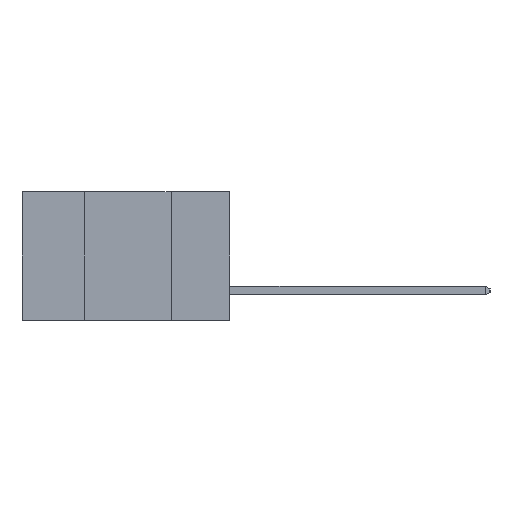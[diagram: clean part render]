
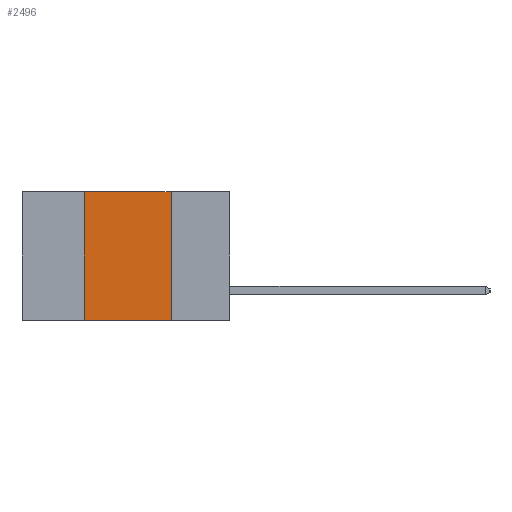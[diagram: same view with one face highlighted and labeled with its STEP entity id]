
A CAD part, left-side view. The second image highlights one B-rep face of the part: STEP entity #2496.
In plain terms, the highlighted planar face has unit normal (-1, 0, 0).
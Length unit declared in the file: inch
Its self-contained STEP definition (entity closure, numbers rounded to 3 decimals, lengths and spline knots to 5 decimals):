
#893 = EDGE_CURVE ( 'NONE', #8158, #3379, #13108, .T. ) ;
#1546 = EDGE_LOOP ( 'NONE', ( #11624, #6986, #12411, #8434 ) ) ;
#1617 = PLANE ( 'NONE',  #4381 ) ;
#1646 = CARTESIAN_POINT ( 'NONE',  ( 0., 0.17, -0.37 ) ) ;
#1681 = CARTESIAN_POINT ( 'NONE',  ( 0., 0.42, -0.37 ) ) ;
#1792 = DIRECTION ( 'NONE',  ( 0., 0., -1. ) ) ;
#2496 = ADVANCED_FACE ( 'NONE', ( #5204 ), #1617, .F. ) ;
#3379 = VERTEX_POINT ( 'NONE', #1646 ) ;
#3680 = EDGE_CURVE ( 'NONE', #8158, #6173, #11944, .T. ) ;
#3730 = VECTOR ( 'NONE', #3761, 39.37008 ) ;
#3753 = VERTEX_POINT ( 'NONE', #12456 ) ;
#3761 = DIRECTION ( 'NONE',  ( 0., 0., 1. ) ) ;
#4220 = CARTESIAN_POINT ( 'NONE',  ( 0., 0.42, 0. ) ) ;
#4381 = AXIS2_PLACEMENT_3D ( 'NONE', #11935, #12851, #1792 ) ;
#5204 = FACE_OUTER_BOUND ( 'NONE', #1546, .T. ) ;
#5396 = CARTESIAN_POINT ( 'NONE',  ( 0., 0.6, -0.37 ) ) ;
#5509 = DIRECTION ( 'NONE',  ( 0., -1., 0. ) ) ;
#6008 = CARTESIAN_POINT ( 'NONE',  ( 0., 0.42, -0.37 ) ) ;
#6173 = VERTEX_POINT ( 'NONE', #4220 ) ;
#6986 = ORIENTED_EDGE ( 'NONE', *, *, #8533, .F. ) ;
#7267 = VECTOR ( 'NONE', #9233, 39.37008 ) ;
#7713 = VECTOR ( 'NONE', #5509, 39.37008 ) ;
#8158 = VERTEX_POINT ( 'NONE', #6008 ) ;
#8434 = ORIENTED_EDGE ( 'NONE', *, *, #893, .T. ) ;
#8533 = EDGE_CURVE ( 'NONE', #6173, #3753, #9899, .T. ) ;
#8678 = CARTESIAN_POINT ( 'NONE',  ( 0., 0.6, 0. ) ) ;
#9233 = DIRECTION ( 'NONE',  ( 0., 0., -1. ) ) ;
#9282 = CARTESIAN_POINT ( 'NONE',  ( 0., 0.17, -0.37 ) ) ;
#9706 = DIRECTION ( 'NONE',  ( 0., -1., 0. ) ) ;
#9899 = LINE ( 'NONE', #8678, #12255 ) ;
#9997 = LINE ( 'NONE', #9282, #7267 ) ;
#11451 = EDGE_CURVE ( 'NONE', #3753, #3379, #9997, .T. ) ;
#11624 = ORIENTED_EDGE ( 'NONE', *, *, #11451, .F. ) ;
#11935 = CARTESIAN_POINT ( 'NONE',  ( 0., 0.6, 0. ) ) ;
#11944 = LINE ( 'NONE', #1681, #3730 ) ;
#12255 = VECTOR ( 'NONE', #9706, 39.37008 ) ;
#12411 = ORIENTED_EDGE ( 'NONE', *, *, #3680, .F. ) ;
#12456 = CARTESIAN_POINT ( 'NONE',  ( 0., 0.17, 0. ) ) ;
#12851 = DIRECTION ( 'NONE',  ( 1., 0., 0. ) ) ;
#13108 = LINE ( 'NONE', #5396, #7713 ) ;
